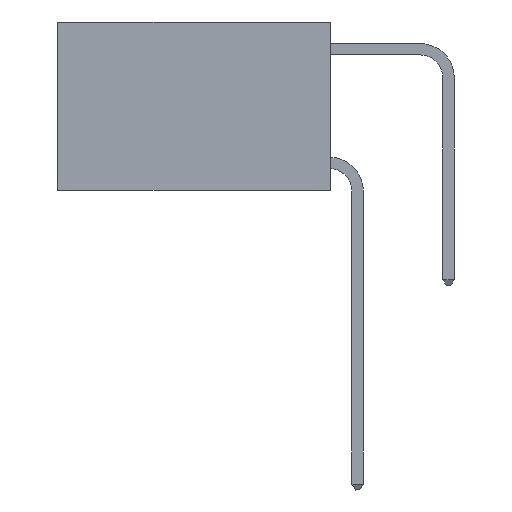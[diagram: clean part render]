
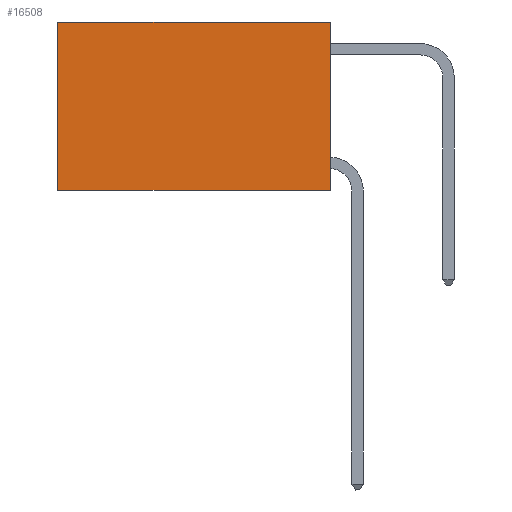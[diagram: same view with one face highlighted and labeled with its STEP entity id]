
A CAD part, left-side view. The second image highlights one B-rep face of the part: STEP entity #16508.
In plain terms, the highlighted planar face has unit normal (-1, 0, 0).
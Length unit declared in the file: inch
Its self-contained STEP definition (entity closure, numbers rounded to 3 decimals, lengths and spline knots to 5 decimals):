
#54 = CARTESIAN_POINT ( 'NONE',  ( 0.2625, 0.6, -0.37 ) ) ;
#274 = CARTESIAN_POINT ( 'NONE',  ( 0.2625, 0.6, 0. ) ) ;
#1375 = DIRECTION ( 'NONE',  ( 1., 0., 0. ) ) ;
#1876 = VERTEX_POINT ( 'NONE', #8618 ) ;
#2092 = LINE ( 'NONE', #274, #14912 ) ;
#2827 = DIRECTION ( 'NONE',  ( 0., 1., 0. ) ) ;
#3734 = ORIENTED_EDGE ( 'NONE', *, *, #18519, .F. ) ;
#3850 = DIRECTION ( 'NONE',  ( 0., 0., -1. ) ) ;
#4806 = CARTESIAN_POINT ( 'NONE',  ( 0.2625, 0., 0. ) ) ;
#7859 = CARTESIAN_POINT ( 'NONE',  ( 0.2625, 0.6, 0. ) ) ;
#8618 = CARTESIAN_POINT ( 'NONE',  ( 0.2625, 0., -0.37 ) ) ;
#10720 = VECTOR ( 'NONE', #14219, 39.37008 ) ;
#11030 = VERTEX_POINT ( 'NONE', #4806 ) ;
#11189 = EDGE_CURVE ( 'NONE', #11030, #29058, #30234, .T. ) ;
#11491 = EDGE_LOOP ( 'NONE', ( #12459, #17591, #3734, #28471 ) ) ;
#12378 = VECTOR ( 'NONE', #2827, 39.37008 ) ;
#12459 = ORIENTED_EDGE ( 'NONE', *, *, #20075, .T. ) ;
#13935 = CARTESIAN_POINT ( 'NONE',  ( 0.2625, 0., -0.37 ) ) ;
#14219 = DIRECTION ( 'NONE',  ( 0., 0., -1. ) ) ;
#14912 = VECTOR ( 'NONE', #27341, 39.37008 ) ;
#15207 = CARTESIAN_POINT ( 'NONE',  ( 0.2625, 0., 0. ) ) ;
#15464 = VECTOR ( 'NONE', #31115, 39.37008 ) ;
#16508 = ADVANCED_FACE ( 'NONE', ( #20861 ), #28309, .F. ) ;
#17591 = ORIENTED_EDGE ( 'NONE', *, *, #29262, .F. ) ;
#18519 = EDGE_CURVE ( 'NONE', #11030, #1876, #29404, .T. ) ;
#19226 = LINE ( 'NONE', #13935, #15464 ) ;
#20075 = EDGE_CURVE ( 'NONE', #29058, #28210, #2092, .T. ) ;
#20861 = FACE_OUTER_BOUND ( 'NONE', #11491, .T. ) ;
#23649 = AXIS2_PLACEMENT_3D ( 'NONE', #26474, #1375, #3850 ) ;
#26474 = CARTESIAN_POINT ( 'NONE',  ( 0.2625, 0., 0. ) ) ;
#27341 = DIRECTION ( 'NONE',  ( 0., 0., -1. ) ) ;
#28210 = VERTEX_POINT ( 'NONE', #54 ) ;
#28309 = PLANE ( 'NONE',  #23649 ) ;
#28471 = ORIENTED_EDGE ( 'NONE', *, *, #11189, .T. ) ;
#29058 = VERTEX_POINT ( 'NONE', #7859 ) ;
#29262 = EDGE_CURVE ( 'NONE', #1876, #28210, #19226, .T. ) ;
#29404 = LINE ( 'NONE', #29722, #10720 ) ;
#29722 = CARTESIAN_POINT ( 'NONE',  ( 0.2625, 0., 0. ) ) ;
#30234 = LINE ( 'NONE', #15207, #12378 ) ;
#31115 = DIRECTION ( 'NONE',  ( 0., 1., 0. ) ) ;
